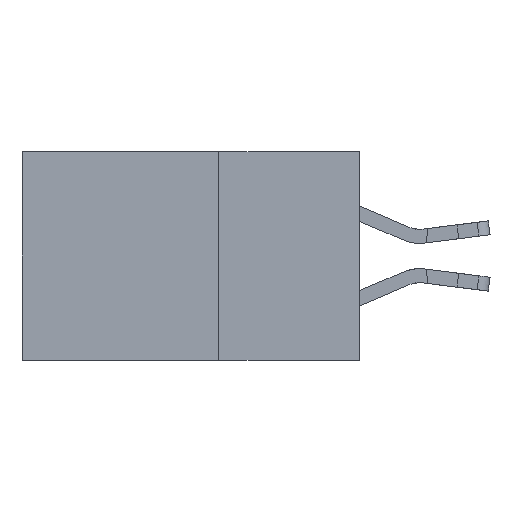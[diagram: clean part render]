
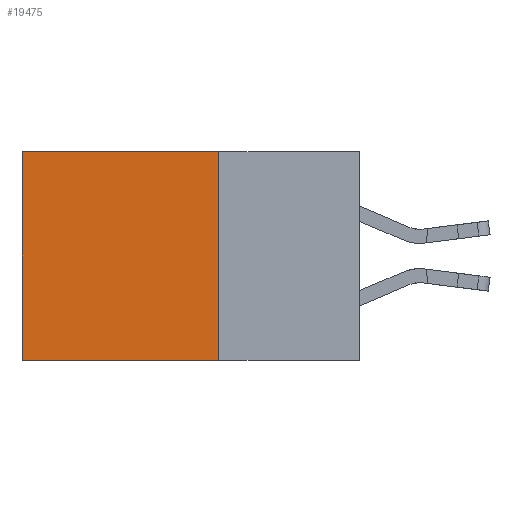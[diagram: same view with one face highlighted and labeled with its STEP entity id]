
A CAD part, left-side view. The second image highlights one B-rep face of the part: STEP entity #19475.
In plain terms, the highlighted planar face has unit normal (-1, 0, 0).
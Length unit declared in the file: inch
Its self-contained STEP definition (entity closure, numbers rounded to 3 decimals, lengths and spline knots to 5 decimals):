
#2781 = ORIENTED_EDGE ( 'NONE', *, *, #20832, .T. ) ;
#2911 = PLANE ( 'NONE',  #5070 ) ;
#2996 = VERTEX_POINT ( 'NONE', #21900 ) ;
#4091 = EDGE_CURVE ( 'NONE', #21540, #2996, #11961, .T. ) ;
#4574 = DIRECTION ( 'NONE',  ( 0., 0., -1. ) ) ;
#5017 = DIRECTION ( 'NONE',  ( 1., 0., 0. ) ) ;
#5070 = AXIS2_PLACEMENT_3D ( 'NONE', #25868, #5017, #4574 ) ;
#5481 = CARTESIAN_POINT ( 'NONE',  ( 0.2875, 0.25, 0. ) ) ;
#6836 = DIRECTION ( 'NONE',  ( 0., 1., 0. ) ) ;
#8353 = CARTESIAN_POINT ( 'NONE',  ( 0.2875, 0.25, -0.37 ) ) ;
#9324 = EDGE_CURVE ( 'NONE', #21540, #18153, #10009, .T. ) ;
#9514 = DIRECTION ( 'NONE',  ( 0., 1., 0. ) ) ;
#10009 = LINE ( 'NONE', #5481, #12563 ) ;
#10298 = CARTESIAN_POINT ( 'NONE',  ( 0.2875, 0.6, 0. ) ) ;
#10314 = DIRECTION ( 'NONE',  ( 0., 0., -1. ) ) ;
#11961 = LINE ( 'NONE', #18927, #16257 ) ;
#12563 = VECTOR ( 'NONE', #10314, 39.37008 ) ;
#12731 = ORIENTED_EDGE ( 'NONE', *, *, #4091, .T. ) ;
#15392 = CARTESIAN_POINT ( 'NONE',  ( 0.2875, 0.25, 0. ) ) ;
#16257 = VECTOR ( 'NONE', #6836, 39.37008 ) ;
#16964 = VERTEX_POINT ( 'NONE', #29732 ) ;
#17306 = ORIENTED_EDGE ( 'NONE', *, *, #9324, .F. ) ;
#18153 = VERTEX_POINT ( 'NONE', #8353 ) ;
#18927 = CARTESIAN_POINT ( 'NONE',  ( 0.2875, 0.25, 0. ) ) ;
#19475 = ADVANCED_FACE ( 'NONE', ( #20887 ), #2911, .F. ) ;
#19752 = VECTOR ( 'NONE', #9514, 39.37008 ) ;
#20050 = ORIENTED_EDGE ( 'NONE', *, *, #28117, .F. ) ;
#20832 = EDGE_CURVE ( 'NONE', #2996, #16964, #29023, .T. ) ;
#20871 = LINE ( 'NONE', #21022, #19752 ) ;
#20887 = FACE_OUTER_BOUND ( 'NONE', #24488, .T. ) ;
#21022 = CARTESIAN_POINT ( 'NONE',  ( 0.2875, 0.25, -0.37 ) ) ;
#21540 = VERTEX_POINT ( 'NONE', #15392 ) ;
#21900 = CARTESIAN_POINT ( 'NONE',  ( 0.2875, 0.6, 0. ) ) ;
#23410 = VECTOR ( 'NONE', #24056, 39.37008 ) ;
#24056 = DIRECTION ( 'NONE',  ( 0., 0., -1. ) ) ;
#24488 = EDGE_LOOP ( 'NONE', ( #2781, #20050, #17306, #12731 ) ) ;
#25868 = CARTESIAN_POINT ( 'NONE',  ( 0.2875, 0.25, 0. ) ) ;
#28117 = EDGE_CURVE ( 'NONE', #18153, #16964, #20871, .T. ) ;
#29023 = LINE ( 'NONE', #10298, #23410 ) ;
#29732 = CARTESIAN_POINT ( 'NONE',  ( 0.2875, 0.6, -0.37 ) ) ;
